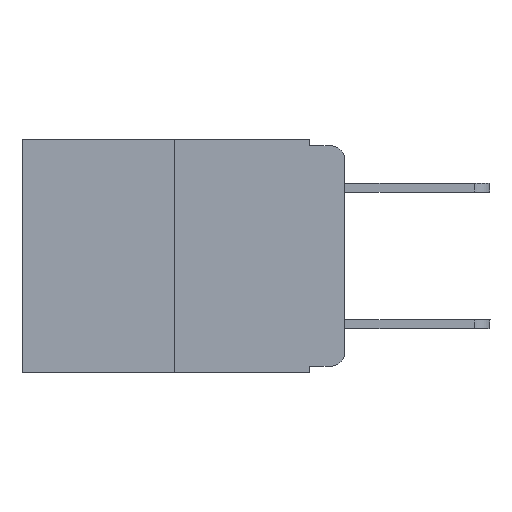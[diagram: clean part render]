
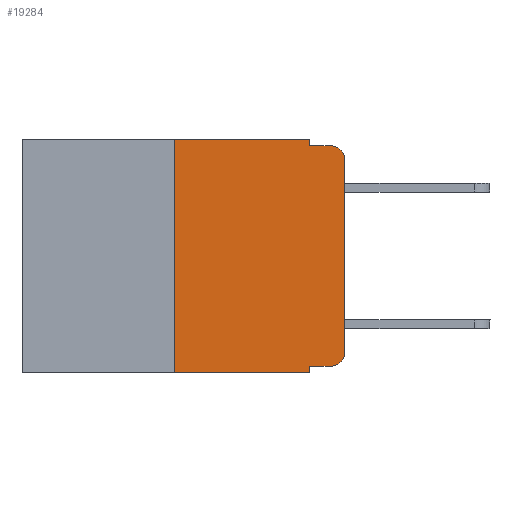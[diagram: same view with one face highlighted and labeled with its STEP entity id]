
A CAD part, left-side view. The second image highlights one B-rep face of the part: STEP entity #19284.
In plain terms, the highlighted planar face has unit normal (-1, 0, 0).
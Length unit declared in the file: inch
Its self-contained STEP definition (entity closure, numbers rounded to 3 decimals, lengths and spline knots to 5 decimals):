
#283 = LINE ( 'NONE', #1073, #8080 ) ;
#1073 = CARTESIAN_POINT ( 'NONE',  ( 0., 0.25, 0. ) ) ;
#1328 = EDGE_CURVE ( 'NONE', #6498, #15390, #3783, .T. ) ;
#1350 = CARTESIAN_POINT ( 'NONE',  ( 0., 0.25, 0. ) ) ;
#1634 = DIRECTION ( 'NONE',  ( 0., 0., -1. ) ) ;
#1694 = ORIENTED_EDGE ( 'NONE', *, *, #1328, .T. ) ;
#1724 = CARTESIAN_POINT ( 'NONE',  ( 0., 0.473, 0. ) ) ;
#1840 = EDGE_CURVE ( 'NONE', #10377, #2285, #14547, .T. ) ;
#1936 = CARTESIAN_POINT ( 'NONE',  ( 0., 0., 0. ) ) ;
#2104 = DIRECTION ( 'NONE',  ( 0., 0., -1. ) ) ;
#2121 = DIRECTION ( 'NONE',  ( 0., -1., 0. ) ) ;
#2285 = VERTEX_POINT ( 'NONE', #17427 ) ;
#2288 = CARTESIAN_POINT ( 'NONE',  ( 0., 0.02, -0.03 ) ) ;
#2327 = ORIENTED_EDGE ( 'NONE', *, *, #6421, .F. ) ;
#2332 = EDGE_CURVE ( 'NONE', #10364, #4268, #5840, .T. ) ;
#2758 = VERTEX_POINT ( 'NONE', #18614 ) ;
#2778 = ORIENTED_EDGE ( 'NONE', *, *, #18193, .F. ) ;
#3259 = ORIENTED_EDGE ( 'NONE', *, *, #18166, .T. ) ;
#3369 = CARTESIAN_POINT ( 'NONE',  ( 0., 0., -0.313 ) ) ;
#3394 = DIRECTION ( 'NONE',  ( 0., 0., -1. ) ) ;
#3783 = CIRCLE ( 'NONE', #9122, 0.02 ) ;
#4113 = VECTOR ( 'NONE', #9521, 39.37008 ) ;
#4268 = VERTEX_POINT ( 'NONE', #10932 ) ;
#4608 = CARTESIAN_POINT ( 'NONE',  ( 0., 0.051, 0. ) ) ;
#4728 = LINE ( 'NONE', #12410, #18082 ) ;
#4987 = VECTOR ( 'NONE', #16471, 39.37008 ) ;
#5442 = FACE_OUTER_BOUND ( 'NONE', #6594, .T. ) ;
#5457 = LINE ( 'NONE', #1936, #16066 ) ;
#5802 = DIRECTION ( 'NONE',  ( 0., 0., -1. ) ) ;
#5840 = LINE ( 'NONE', #6060, #4113 ) ;
#6060 = CARTESIAN_POINT ( 'NONE',  ( 0., 0.473, -0.343 ) ) ;
#6235 = LINE ( 'NONE', #19190, #10032 ) ;
#6421 = EDGE_CURVE ( 'NONE', #9513, #4268, #4728, .T. ) ;
#6498 = VERTEX_POINT ( 'NONE', #12356 ) ;
#6594 = EDGE_LOOP ( 'NONE', ( #3259, #1694, #2778, #20596, #8137, #18394, #19665, #2327, #19360, #12505 ) ) ;
#6964 = EDGE_CURVE ( 'NONE', #2758, #10971, #12496, .T. ) ;
#7721 = LINE ( 'NONE', #1724, #11513 ) ;
#8080 = VECTOR ( 'NONE', #15511, 39.37008 ) ;
#8137 = ORIENTED_EDGE ( 'NONE', *, *, #19688, .F. ) ;
#8215 = CARTESIAN_POINT ( 'NONE',  ( 0., 0.051, 0. ) ) ;
#8245 = CARTESIAN_POINT ( 'NONE',  ( 0., 0.051, -0.01 ) ) ;
#8463 = DIRECTION ( 'NONE',  ( -1., 0., 0. ) ) ;
#8773 = AXIS2_PLACEMENT_3D ( 'NONE', #15386, #8979, #5802 ) ;
#8979 = DIRECTION ( 'NONE',  ( -1., 0., 0. ) ) ;
#9122 = AXIS2_PLACEMENT_3D ( 'NONE', #2288, #8463, #2104 ) ;
#9504 = DIRECTION ( 'NONE',  ( 0., -1., 0. ) ) ;
#9513 = VERTEX_POINT ( 'NONE', #19919 ) ;
#9521 = DIRECTION ( 'NONE',  ( 0., -1., 0. ) ) ;
#9630 = PLANE ( 'NONE',  #11107 ) ;
#10032 = VECTOR ( 'NONE', #9504, 39.37008 ) ;
#10290 = VECTOR ( 'NONE', #3394, 39.37008 ) ;
#10364 = VERTEX_POINT ( 'NONE', #11476 ) ;
#10377 = VERTEX_POINT ( 'NONE', #8215 ) ;
#10932 = CARTESIAN_POINT ( 'NONE',  ( 0., 0.051, -0.343 ) ) ;
#10971 = VERTEX_POINT ( 'NONE', #3369 ) ;
#11107 = AXIS2_PLACEMENT_3D ( 'NONE', #17762, #16303, #1634 ) ;
#11476 = CARTESIAN_POINT ( 'NONE',  ( 0., 0.25, -0.343 ) ) ;
#11513 = VECTOR ( 'NONE', #2121, 39.37008 ) ;
#11531 = LINE ( 'NONE', #8245, #4987 ) ;
#12356 = CARTESIAN_POINT ( 'NONE',  ( 0., 0., -0.03 ) ) ;
#12410 = CARTESIAN_POINT ( 'NONE',  ( 0., 0.051, 0. ) ) ;
#12496 = CIRCLE ( 'NONE', #8773, 0.02 ) ;
#12505 = ORIENTED_EDGE ( 'NONE', *, *, #6964, .T. ) ;
#12535 = EDGE_CURVE ( 'NONE', #9513, #2758, #6235, .T. ) ;
#14547 = LINE ( 'NONE', #4608, #10290 ) ;
#14688 = VERTEX_POINT ( 'NONE', #1350 ) ;
#15386 = CARTESIAN_POINT ( 'NONE',  ( 0., 0.02, -0.313 ) ) ;
#15390 = VERTEX_POINT ( 'NONE', #17487 ) ;
#15511 = DIRECTION ( 'NONE',  ( 0., 0., 1. ) ) ;
#16066 = VECTOR ( 'NONE', #16403, 39.37008 ) ;
#16303 = DIRECTION ( 'NONE',  ( 1., 0., 0. ) ) ;
#16358 = EDGE_CURVE ( 'NONE', #10364, #14688, #283, .T. ) ;
#16403 = DIRECTION ( 'NONE',  ( 0., 0., 1. ) ) ;
#16471 = DIRECTION ( 'NONE',  ( 0., -1., 0. ) ) ;
#17427 = CARTESIAN_POINT ( 'NONE',  ( 0., 0.051, -0.01 ) ) ;
#17487 = CARTESIAN_POINT ( 'NONE',  ( 0., 0.02, -0.01 ) ) ;
#17542 = DIRECTION ( 'NONE',  ( 0., 0., -1. ) ) ;
#17762 = CARTESIAN_POINT ( 'NONE',  ( 0., 0.473, 0. ) ) ;
#18082 = VECTOR ( 'NONE', #17542, 39.37008 ) ;
#18166 = EDGE_CURVE ( 'NONE', #10971, #6498, #5457, .T. ) ;
#18193 = EDGE_CURVE ( 'NONE', #2285, #15390, #11531, .T. ) ;
#18394 = ORIENTED_EDGE ( 'NONE', *, *, #16358, .F. ) ;
#18614 = CARTESIAN_POINT ( 'NONE',  ( 0., 0.02, -0.333 ) ) ;
#19190 = CARTESIAN_POINT ( 'NONE',  ( 0., 0.051, -0.333 ) ) ;
#19284 = ADVANCED_FACE ( 'NONE', ( #5442 ), #9630, .F. ) ;
#19360 = ORIENTED_EDGE ( 'NONE', *, *, #12535, .T. ) ;
#19665 = ORIENTED_EDGE ( 'NONE', *, *, #2332, .T. ) ;
#19688 = EDGE_CURVE ( 'NONE', #14688, #10377, #7721, .T. ) ;
#19919 = CARTESIAN_POINT ( 'NONE',  ( 0., 0.051, -0.333 ) ) ;
#20596 = ORIENTED_EDGE ( 'NONE', *, *, #1840, .F. ) ;
